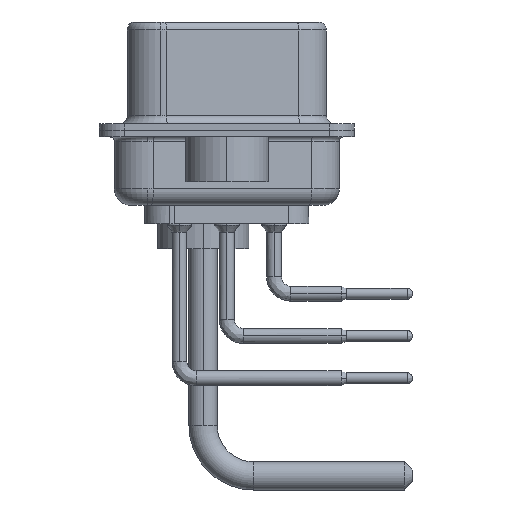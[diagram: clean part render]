
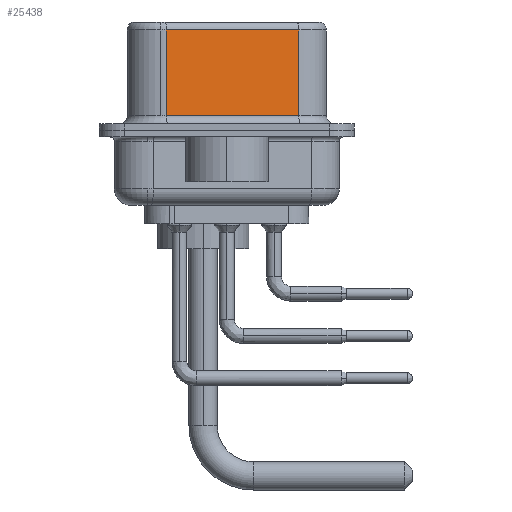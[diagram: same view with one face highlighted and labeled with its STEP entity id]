
A CAD part, left-side view. The second image highlights one B-rep face of the part: STEP entity #25438.
In plain terms, the highlighted planar face has unit normal (-0.985, -0.174, 0).
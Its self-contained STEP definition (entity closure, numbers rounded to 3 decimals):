
#350 = VECTOR ( 'NONE', #461, 1000. ) ;
#461 = DIRECTION ( 'NONE',  ( -0.174, 0.985, 0. ) ) ;
#941 = ORIENTED_EDGE ( 'NONE', *, *, #23435, .T. ) ;
#1125 = LINE ( 'NONE', #31655, #29866 ) ;
#1294 = CARTESIAN_POINT ( 'NONE',  ( 5.132, -4.322, 0.9 ) ) ;
#3992 = ORIENTED_EDGE ( 'NONE', *, *, #25398, .T. ) ;
#4755 = CARTESIAN_POINT ( 'NONE',  ( 3.73, 3.628, 6.52 ) ) ;
#5108 = DIRECTION ( 'NONE',  ( -0.174, 0.985, 0. ) ) ;
#5251 = EDGE_CURVE ( 'NONE', #13255, #29093, #33708, .T. ) ;
#6135 = LINE ( 'NONE', #26384, #350 ) ;
#6487 = CARTESIAN_POINT ( 'NONE',  ( 5.132, -4.322, 6.02 ) ) ;
#8198 = CARTESIAN_POINT ( 'NONE',  ( 3.73, 3.628, 0.9 ) ) ;
#8711 = VECTOR ( 'NONE', #13452, 1000. ) ;
#9891 = VERTEX_POINT ( 'NONE', #1294 ) ;
#10623 = CARTESIAN_POINT ( 'NONE',  ( 5.132, -4.322, 6.52 ) ) ;
#11020 = EDGE_CURVE ( 'NONE', #27401, #9891, #1125, .T. ) ;
#12206 = VECTOR ( 'NONE', #19522, 1000. ) ;
#12291 = CARTESIAN_POINT ( 'NONE',  ( 3.73, 3.628, 6.02 ) ) ;
#13255 = VERTEX_POINT ( 'NONE', #12291 ) ;
#13452 = DIRECTION ( 'NONE',  ( 0.174, -0.985, 0. ) ) ;
#13659 = FACE_OUTER_BOUND ( 'NONE', #20006, .T. ) ;
#19487 = CARTESIAN_POINT ( 'NONE',  ( 5.132, -4.322, 0.9 ) ) ;
#19522 = DIRECTION ( 'NONE',  ( 0., 0., -1. ) ) ;
#20006 = EDGE_LOOP ( 'NONE', ( #29307, #941, #34122, #3992 ) ) ;
#23133 = DIRECTION ( 'NONE',  ( 0., 0., -1. ) ) ;
#23435 = EDGE_CURVE ( 'NONE', #27401, #13255, #6135, .T. ) ;
#24780 = DIRECTION ( 'NONE',  ( 0.985, 0.174, 0. ) ) ;
#24993 = AXIS2_PLACEMENT_3D ( 'NONE', #10623, #24780, #5108 ) ;
#25398 = EDGE_CURVE ( 'NONE', #29093, #9891, #36339, .T. ) ;
#25438 = ADVANCED_FACE ( 'NONE', ( #13659 ), #36735, .F. ) ;
#26384 = CARTESIAN_POINT ( 'NONE',  ( 5.132, -4.322, 6.02 ) ) ;
#27401 = VERTEX_POINT ( 'NONE', #6487 ) ;
#29093 = VERTEX_POINT ( 'NONE', #8198 ) ;
#29307 = ORIENTED_EDGE ( 'NONE', *, *, #11020, .F. ) ;
#29866 = VECTOR ( 'NONE', #23133, 1000. ) ;
#31655 = CARTESIAN_POINT ( 'NONE',  ( 5.132, -4.322, 6.52 ) ) ;
#33708 = LINE ( 'NONE', #4755, #12206 ) ;
#34122 = ORIENTED_EDGE ( 'NONE', *, *, #5251, .T. ) ;
#36339 = LINE ( 'NONE', #19487, #8711 ) ;
#36735 = PLANE ( 'NONE',  #24993 ) ;
